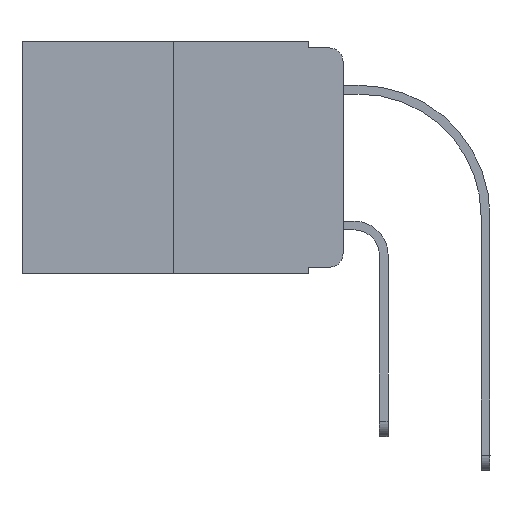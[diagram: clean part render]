
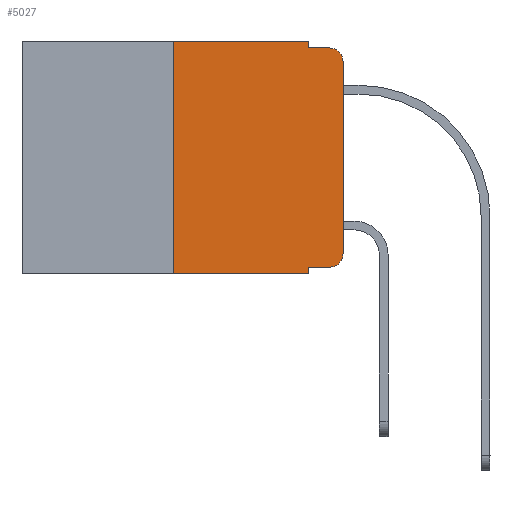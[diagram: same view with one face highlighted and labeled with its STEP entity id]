
A CAD part, left-side view. The second image highlights one B-rep face of the part: STEP entity #5027.
In plain terms, the highlighted planar face has unit normal (-1, 0, 0).
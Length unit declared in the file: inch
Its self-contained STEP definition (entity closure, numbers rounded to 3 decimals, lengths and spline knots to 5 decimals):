
#395 = EDGE_CURVE ( 'NONE', #13945, #1709, #8960, .T. ) ;
#427 = CARTESIAN_POINT ( 'NONE',  ( 0., 0.473, 0. ) ) ;
#550 = VECTOR ( 'NONE', #11211, 39.37008 ) ;
#849 = VERTEX_POINT ( 'NONE', #10037 ) ;
#1058 = VERTEX_POINT ( 'NONE', #11077 ) ;
#1107 = CARTESIAN_POINT ( 'NONE',  ( 0., 0.25, 0. ) ) ;
#1590 = CARTESIAN_POINT ( 'NONE',  ( 0., 0.051, 0. ) ) ;
#1675 = CIRCLE ( 'NONE', #12590, 0.02 ) ;
#1709 = VERTEX_POINT ( 'NONE', #13082 ) ;
#1770 = VERTEX_POINT ( 'NONE', #14939 ) ;
#1877 = LINE ( 'NONE', #4813, #7578 ) ;
#1955 = ORIENTED_EDGE ( 'NONE', *, *, #6713, .T. ) ;
#2141 = DIRECTION ( 'NONE',  ( -1., 0., 0. ) ) ;
#2424 = DIRECTION ( 'NONE',  ( 1., 0., 0. ) ) ;
#2637 = ORIENTED_EDGE ( 'NONE', *, *, #17588, .T. ) ;
#2815 = ORIENTED_EDGE ( 'NONE', *, *, #11326, .F. ) ;
#2966 = ORIENTED_EDGE ( 'NONE', *, *, #7723, .F. ) ;
#3483 = ORIENTED_EDGE ( 'NONE', *, *, #11981, .F. ) ;
#3542 = CARTESIAN_POINT ( 'NONE',  ( 0., 0.051, 0. ) ) ;
#3772 = EDGE_CURVE ( 'NONE', #849, #15054, #1675, .T. ) ;
#4813 = CARTESIAN_POINT ( 'NONE',  ( 0., 0.051, -0.01 ) ) ;
#4836 = LINE ( 'NONE', #6011, #5972 ) ;
#5027 = ADVANCED_FACE ( 'NONE', ( #15912 ), #18643, .F. ) ;
#5551 = DIRECTION ( 'NONE',  ( 0., 0., -1. ) ) ;
#5944 = CIRCLE ( 'NONE', #8115, 0.02 ) ;
#5972 = VECTOR ( 'NONE', #18021, 39.37008 ) ;
#6011 = CARTESIAN_POINT ( 'NONE',  ( 0., 0.473, -0.343 ) ) ;
#6452 = CARTESIAN_POINT ( 'NONE',  ( 0., 0.02, -0.03 ) ) ;
#6569 = LINE ( 'NONE', #3542, #9597 ) ;
#6645 = DIRECTION ( 'NONE',  ( 0., 0., -1. ) ) ;
#6713 = EDGE_CURVE ( 'NONE', #15054, #1770, #13747, .T. ) ;
#6735 = DIRECTION ( 'NONE',  ( -1., 0., 0. ) ) ;
#7015 = CARTESIAN_POINT ( 'NONE',  ( 0., 0.473, 0. ) ) ;
#7314 = CARTESIAN_POINT ( 'NONE',  ( 0., 0.051, 0. ) ) ;
#7578 = VECTOR ( 'NONE', #18098, 39.37008 ) ;
#7723 = EDGE_CURVE ( 'NONE', #12306, #1058, #6569, .T. ) ;
#7839 = DIRECTION ( 'NONE',  ( 0., -1., 0. ) ) ;
#7966 = CARTESIAN_POINT ( 'NONE',  ( 0., 0.25, 0. ) ) ;
#8115 = AXIS2_PLACEMENT_3D ( 'NONE', #6452, #6735, #6645 ) ;
#8446 = EDGE_LOOP ( 'NONE', ( #1955, #9205, #2815, #2966, #3483, #14922, #2637, #11926, #19277, #15070 ) ) ;
#8960 = LINE ( 'NONE', #7314, #16520 ) ;
#9205 = ORIENTED_EDGE ( 'NONE', *, *, #10299, .T. ) ;
#9597 = VECTOR ( 'NONE', #13890, 39.37008 ) ;
#9653 = DIRECTION ( 'NONE',  ( 0., 0., -1. ) ) ;
#9780 = CARTESIAN_POINT ( 'NONE',  ( 0., 0.051, -0.333 ) ) ;
#10037 = CARTESIAN_POINT ( 'NONE',  ( 0., 0.02, -0.333 ) ) ;
#10299 = EDGE_CURVE ( 'NONE', #1770, #16525, #5944, .T. ) ;
#10317 = CARTESIAN_POINT ( 'NONE',  ( 0., 0., -0.313 ) ) ;
#11077 = CARTESIAN_POINT ( 'NONE',  ( 0., 0.051, -0.01 ) ) ;
#11211 = DIRECTION ( 'NONE',  ( 0., -1., 0. ) ) ;
#11281 = DIRECTION ( 'NONE',  ( 0., 0., 1. ) ) ;
#11326 = EDGE_CURVE ( 'NONE', #1058, #16525, #1877, .T. ) ;
#11403 = LINE ( 'NONE', #17360, #550 ) ;
#11926 = ORIENTED_EDGE ( 'NONE', *, *, #395, .F. ) ;
#11981 = EDGE_CURVE ( 'NONE', #19224, #12306, #17123, .T. ) ;
#12126 = CARTESIAN_POINT ( 'NONE',  ( 0., 0.25, -0.343 ) ) ;
#12274 = DIRECTION ( 'NONE',  ( 0., 0., 1. ) ) ;
#12306 = VERTEX_POINT ( 'NONE', #1590 ) ;
#12590 = AXIS2_PLACEMENT_3D ( 'NONE', #13662, #2141, #9653 ) ;
#13057 = EDGE_CURVE ( 'NONE', #13945, #849, #11403, .T. ) ;
#13082 = CARTESIAN_POINT ( 'NONE',  ( 0., 0.051, -0.343 ) ) ;
#13611 = VERTEX_POINT ( 'NONE', #12126 ) ;
#13662 = CARTESIAN_POINT ( 'NONE',  ( 0., 0.02, -0.313 ) ) ;
#13747 = LINE ( 'NONE', #18341, #17358 ) ;
#13890 = DIRECTION ( 'NONE',  ( 0., 0., -1. ) ) ;
#13945 = VERTEX_POINT ( 'NONE', #9780 ) ;
#14744 = DIRECTION ( 'NONE',  ( 0., 0., -1. ) ) ;
#14922 = ORIENTED_EDGE ( 'NONE', *, *, #17352, .F. ) ;
#14939 = CARTESIAN_POINT ( 'NONE',  ( 0., 0., -0.03 ) ) ;
#15054 = VERTEX_POINT ( 'NONE', #10317 ) ;
#15070 = ORIENTED_EDGE ( 'NONE', *, *, #3772, .T. ) ;
#15171 = VECTOR ( 'NONE', #7839, 39.37008 ) ;
#15912 = FACE_OUTER_BOUND ( 'NONE', #8446, .T. ) ;
#15958 = CARTESIAN_POINT ( 'NONE',  ( 0., 0.02, -0.01 ) ) ;
#16520 = VECTOR ( 'NONE', #14744, 39.37008 ) ;
#16525 = VERTEX_POINT ( 'NONE', #15958 ) ;
#17051 = LINE ( 'NONE', #7966, #18129 ) ;
#17123 = LINE ( 'NONE', #427, #15171 ) ;
#17352 = EDGE_CURVE ( 'NONE', #13611, #19224, #17051, .T. ) ;
#17358 = VECTOR ( 'NONE', #12274, 39.37008 ) ;
#17360 = CARTESIAN_POINT ( 'NONE',  ( 0., 0.051, -0.333 ) ) ;
#17588 = EDGE_CURVE ( 'NONE', #13611, #1709, #4836, .T. ) ;
#18021 = DIRECTION ( 'NONE',  ( 0., -1., 0. ) ) ;
#18098 = DIRECTION ( 'NONE',  ( 0., -1., 0. ) ) ;
#18129 = VECTOR ( 'NONE', #11281, 39.37008 ) ;
#18242 = AXIS2_PLACEMENT_3D ( 'NONE', #7015, #2424, #5551 ) ;
#18341 = CARTESIAN_POINT ( 'NONE',  ( 0., 0., 0. ) ) ;
#18643 = PLANE ( 'NONE',  #18242 ) ;
#19224 = VERTEX_POINT ( 'NONE', #1107 ) ;
#19277 = ORIENTED_EDGE ( 'NONE', *, *, #13057, .T. ) ;
